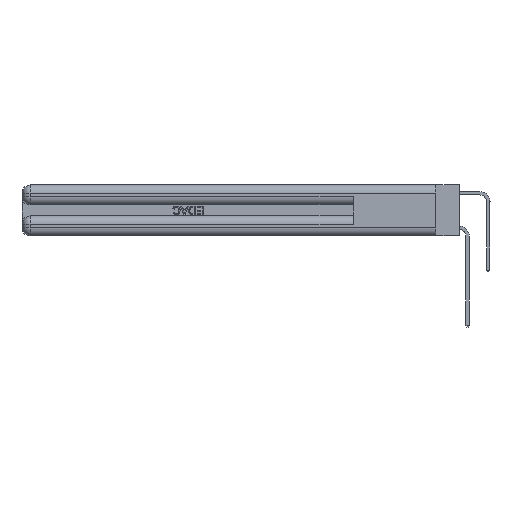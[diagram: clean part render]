
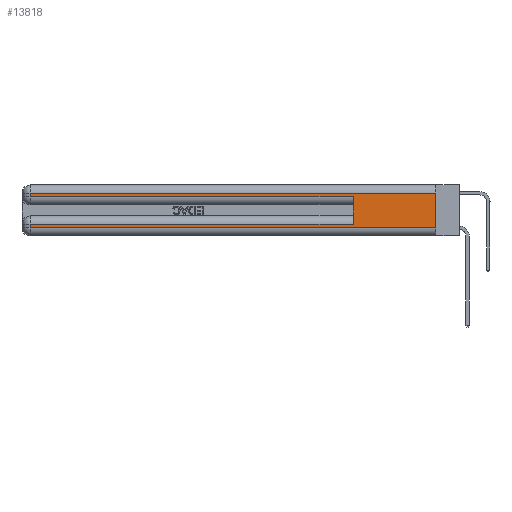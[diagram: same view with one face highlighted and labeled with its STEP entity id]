
A CAD part, left-side view. The second image highlights one B-rep face of the part: STEP entity #13818.
In plain terms, the highlighted planar face has unit normal (-1, 0, 0).
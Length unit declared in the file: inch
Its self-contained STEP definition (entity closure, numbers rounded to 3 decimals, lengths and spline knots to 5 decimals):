
#447 = CARTESIAN_POINT ( 'NONE',  ( 0., 0., 0.37 ) ) ;
#767 = DIRECTION ( 'NONE',  ( 0., 1., 0. ) ) ;
#988 = CARTESIAN_POINT ( 'NONE',  ( 0., 2.94, 0.37 ) ) ;
#1033 = PLANE ( 'NONE',  #7292 ) ;
#1372 = CARTESIAN_POINT ( 'NONE',  ( 0., 0.6, 0.145 ) ) ;
#1811 = VERTEX_POINT ( 'NONE', #5394 ) ;
#2263 = DIRECTION ( 'NONE',  ( 0., -1., 0. ) ) ;
#2737 = ORIENTED_EDGE ( 'NONE', *, *, #15912, .T. ) ;
#2900 = CARTESIAN_POINT ( 'NONE',  ( 0., 0., 0.285 ) ) ;
#3256 = CARTESIAN_POINT ( 'NONE',  ( 0., 0., 0.085 ) ) ;
#3719 = EDGE_CURVE ( 'NONE', #10198, #10616, #24469, .T. ) ;
#3929 = ORIENTED_EDGE ( 'NONE', *, *, #14913, .T. ) ;
#4907 = VECTOR ( 'NONE', #27400, 39.37008 ) ;
#5037 = VECTOR ( 'NONE', #19016, 39.37008 ) ;
#5394 = CARTESIAN_POINT ( 'NONE',  ( 0., 0.6, 0.085 ) ) ;
#5720 = VERTEX_POINT ( 'NONE', #12612 ) ;
#6647 = EDGE_CURVE ( 'NONE', #27660, #10198, #35229, .T. ) ;
#7292 = AXIS2_PLACEMENT_3D ( 'NONE', #31502, #12219, #25821 ) ;
#7744 = CARTESIAN_POINT ( 'NONE',  ( 0., 2.94, 0.37 ) ) ;
#8721 = DIRECTION ( 'NONE',  ( 0., 0., -1. ) ) ;
#8865 = ORIENTED_EDGE ( 'NONE', *, *, #3719, .T. ) ;
#8906 = CARTESIAN_POINT ( 'NONE',  ( 0., 0.6, 0.285 ) ) ;
#9280 = VECTOR ( 'NONE', #2263, 39.37008 ) ;
#9713 = CARTESIAN_POINT ( 'NONE',  ( 0., 0., 0.06 ) ) ;
#9893 = CARTESIAN_POINT ( 'NONE',  ( 0., 2.94, 0.06 ) ) ;
#10198 = VERTEX_POINT ( 'NONE', #33693 ) ;
#10616 = VERTEX_POINT ( 'NONE', #16757 ) ;
#11328 = VERTEX_POINT ( 'NONE', #9713 ) ;
#12219 = DIRECTION ( 'NONE',  ( 1., 0., 0. ) ) ;
#12612 = CARTESIAN_POINT ( 'NONE',  ( 0., 2.94, 0.085 ) ) ;
#13207 = VECTOR ( 'NONE', #35495, 39.37008 ) ;
#13241 = CARTESIAN_POINT ( 'NONE',  ( 0., 0., 0.31 ) ) ;
#13818 = ADVANCED_FACE ( 'NONE', ( #23547 ), #1033, .F. ) ;
#14347 = EDGE_LOOP ( 'NONE', ( #18151, #32612, #8865, #2737, #14835, #20405, #20224, #3929 ) ) ;
#14443 = EDGE_CURVE ( 'NONE', #1811, #5720, #26930, .T. ) ;
#14835 = ORIENTED_EDGE ( 'NONE', *, *, #19769, .F. ) ;
#14913 = EDGE_CURVE ( 'NONE', #15186, #11328, #16597, .T. ) ;
#15186 = VERTEX_POINT ( 'NONE', #9893 ) ;
#15912 = EDGE_CURVE ( 'NONE', #10616, #21782, #17385, .T. ) ;
#16597 = LINE ( 'NONE', #19015, #9280 ) ;
#16757 = CARTESIAN_POINT ( 'NONE',  ( 0., 2.94, 0.285 ) ) ;
#17385 = LINE ( 'NONE', #2900, #4907 ) ;
#17584 = VECTOR ( 'NONE', #19783, 39.37008 ) ;
#18151 = ORIENTED_EDGE ( 'NONE', *, *, #30576, .F. ) ;
#19015 = CARTESIAN_POINT ( 'NONE',  ( 0., 0., 0.06 ) ) ;
#19016 = DIRECTION ( 'NONE',  ( 0., 0., -1. ) ) ;
#19164 = CARTESIAN_POINT ( 'NONE',  ( 0., 0., 0.31 ) ) ;
#19769 = EDGE_CURVE ( 'NONE', #1811, #21782, #28972, .T. ) ;
#19783 = DIRECTION ( 'NONE',  ( 0., 0., -1. ) ) ;
#20224 = ORIENTED_EDGE ( 'NONE', *, *, #23930, .T. ) ;
#20405 = ORIENTED_EDGE ( 'NONE', *, *, #14443, .T. ) ;
#21782 = VERTEX_POINT ( 'NONE', #8906 ) ;
#22677 = LINE ( 'NONE', #7744, #5037 ) ;
#22912 = VECTOR ( 'NONE', #31261, 39.37008 ) ;
#23547 = FACE_OUTER_BOUND ( 'NONE', #14347, .T. ) ;
#23930 = EDGE_CURVE ( 'NONE', #5720, #15186, #22677, .T. ) ;
#24469 = LINE ( 'NONE', #988, #27109 ) ;
#25821 = DIRECTION ( 'NONE',  ( 0., 0., -1. ) ) ;
#26930 = LINE ( 'NONE', #3256, #33013 ) ;
#27109 = VECTOR ( 'NONE', #8721, 39.37008 ) ;
#27400 = DIRECTION ( 'NONE',  ( 0., -1., 0. ) ) ;
#27660 = VERTEX_POINT ( 'NONE', #13241 ) ;
#28972 = LINE ( 'NONE', #1372, #22912 ) ;
#30576 = EDGE_CURVE ( 'NONE', #27660, #11328, #31371, .T. ) ;
#31261 = DIRECTION ( 'NONE',  ( 0., 0., 1. ) ) ;
#31371 = LINE ( 'NONE', #447, #17584 ) ;
#31502 = CARTESIAN_POINT ( 'NONE',  ( 0., 0., 0.37 ) ) ;
#32612 = ORIENTED_EDGE ( 'NONE', *, *, #6647, .T. ) ;
#33013 = VECTOR ( 'NONE', #767, 39.37008 ) ;
#33693 = CARTESIAN_POINT ( 'NONE',  ( 0., 2.94, 0.31 ) ) ;
#35229 = LINE ( 'NONE', #19164, #13207 ) ;
#35495 = DIRECTION ( 'NONE',  ( 0., 1., 0. ) ) ;
